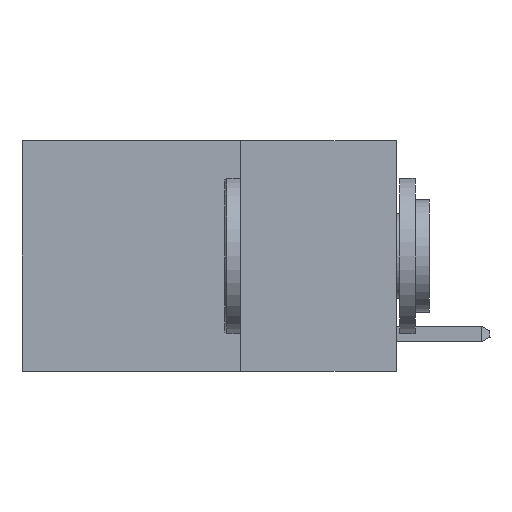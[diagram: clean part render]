
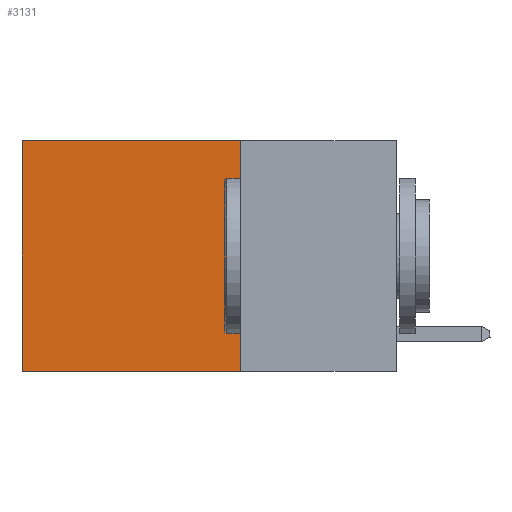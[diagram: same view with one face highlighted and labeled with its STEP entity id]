
A CAD part, left-side view. The second image highlights one B-rep face of the part: STEP entity #3131.
In plain terms, the highlighted planar face has unit normal (-1, 0, 0).
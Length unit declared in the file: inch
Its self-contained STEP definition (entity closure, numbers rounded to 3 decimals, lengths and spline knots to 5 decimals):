
#7 = VERTEX_POINT ( 'NONE', #5894 ) ;
#248 = ORIENTED_EDGE ( 'NONE', *, *, #5097, .T. ) ;
#273 = LINE ( 'NONE', #10170, #13582 ) ;
#455 = VERTEX_POINT ( 'NONE', #13058 ) ;
#1190 = AXIS2_PLACEMENT_3D ( 'NONE', #8424, #9747, #1982 ) ;
#1430 = DIRECTION ( 'NONE',  ( 0., 0., -1. ) ) ;
#1982 = DIRECTION ( 'NONE',  ( 0., 0., -1. ) ) ;
#2139 = EDGE_LOOP ( 'NONE', ( #248, #9997, #7734, #13488 ) ) ;
#2691 = EDGE_CURVE ( 'NONE', #455, #14415, #273, .T. ) ;
#3121 = VECTOR ( 'NONE', #10760, 39.37008 ) ;
#3131 = ADVANCED_FACE ( 'NONE', ( #4100 ), #15950, .F. ) ;
#3465 = LINE ( 'NONE', #5237, #16544 ) ;
#3831 = VERTEX_POINT ( 'NONE', #8516 ) ;
#4100 = FACE_OUTER_BOUND ( 'NONE', #2139, .T. ) ;
#5097 = EDGE_CURVE ( 'NONE', #7, #3831, #3465, .T. ) ;
#5237 = CARTESIAN_POINT ( 'NONE',  ( 0.2625, 0.6, 0. ) ) ;
#5894 = CARTESIAN_POINT ( 'NONE',  ( 0.2625, 0.6, 0. ) ) ;
#5934 = EDGE_CURVE ( 'NONE', #14415, #3831, #8892, .T. ) ;
#6258 = DIRECTION ( 'NONE',  ( 0., 0., -1. ) ) ;
#6487 = CARTESIAN_POINT ( 'NONE',  ( 0.2625, 0.25, -0.37 ) ) ;
#6509 = LINE ( 'NONE', #15656, #3121 ) ;
#7246 = EDGE_CURVE ( 'NONE', #455, #7, #6509, .T. ) ;
#7734 = ORIENTED_EDGE ( 'NONE', *, *, #2691, .F. ) ;
#8424 = CARTESIAN_POINT ( 'NONE',  ( 0.2625, 0.25, 0. ) ) ;
#8516 = CARTESIAN_POINT ( 'NONE',  ( 0.2625, 0.6, -0.37 ) ) ;
#8892 = LINE ( 'NONE', #12526, #15178 ) ;
#9747 = DIRECTION ( 'NONE',  ( 1., 0., 0. ) ) ;
#9997 = ORIENTED_EDGE ( 'NONE', *, *, #5934, .F. ) ;
#10170 = CARTESIAN_POINT ( 'NONE',  ( 0.2625, 0.25, 0. ) ) ;
#10760 = DIRECTION ( 'NONE',  ( 0., 1., 0. ) ) ;
#12526 = CARTESIAN_POINT ( 'NONE',  ( 0.2625, 0.25, -0.37 ) ) ;
#13058 = CARTESIAN_POINT ( 'NONE',  ( 0.2625, 0.25, 0. ) ) ;
#13488 = ORIENTED_EDGE ( 'NONE', *, *, #7246, .T. ) ;
#13582 = VECTOR ( 'NONE', #6258, 39.37008 ) ;
#13762 = DIRECTION ( 'NONE',  ( 0., 1., 0. ) ) ;
#14415 = VERTEX_POINT ( 'NONE', #6487 ) ;
#15178 = VECTOR ( 'NONE', #13762, 39.37008 ) ;
#15656 = CARTESIAN_POINT ( 'NONE',  ( 0.2625, 0.25, 0. ) ) ;
#15950 = PLANE ( 'NONE',  #1190 ) ;
#16544 = VECTOR ( 'NONE', #1430, 39.37008 ) ;
